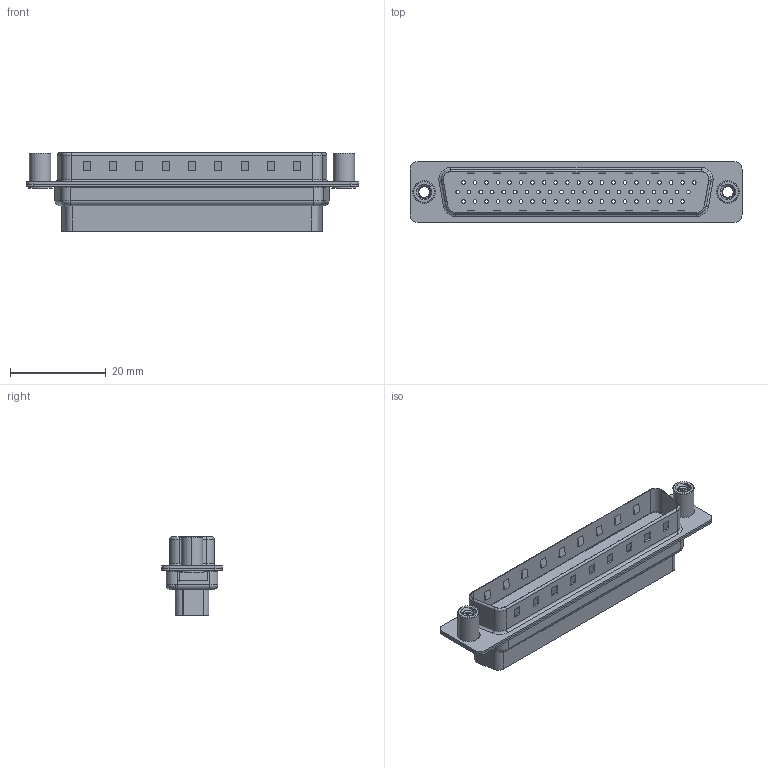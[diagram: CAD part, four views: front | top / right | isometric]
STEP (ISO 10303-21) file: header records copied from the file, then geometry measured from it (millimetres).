
FILE_DESCRIPTION (( 'STEP AP203' ), '1' );
FILE_NAME ('637-062-010-048.STEP', '2020-07-17T21:26:16', ( '' ), ( '' ), 'SwSTEP 2.0', 'SolidWorks 2020', '' );
FILE_SCHEMA (( 'CONFIG_CONTROL_DESIGN' ));
Length unit declared in the file: millimetre
Products named in the file (5): 637-062-010-048; 637 Shell Front_62 Contacts; 637 4-40 Threaded Standoff; 637 Shell Rear_62 Contacts; 637 Housing_62 Contacts HP
Assembly tree (5 placements, depth 2):
  637-062-010-048
    637 Housing_62 Contacts HP
    637 Shell Front_62 Contacts
    637 Shell Rear_62 Contacts
    637 4-40 Threaded Standoff  x2
Bounding box: 69.4 x 12.6 x 16.4 mm (x, y, z)
Volume: 4220.6 mm3; surface area: 9987.1 mm2
Topology: 5 solids, 5 shells, 942 faces, 2265 edges, 1470 vertices
Faces by surface type: cylinder 541, plane 329, torus 50, cone 16, bspline 6
Entity records: 28739 total; most frequent: CARTESIAN_POINT 6247, DIRECTION 4908, ORIENTED_EDGE 4276, EDGE_CURVE 2138, AXIS2_PLACEMENT_3D 1944, VERTEX_POINT 1388, EDGE_LOOP 1200, CIRCLE 1047
